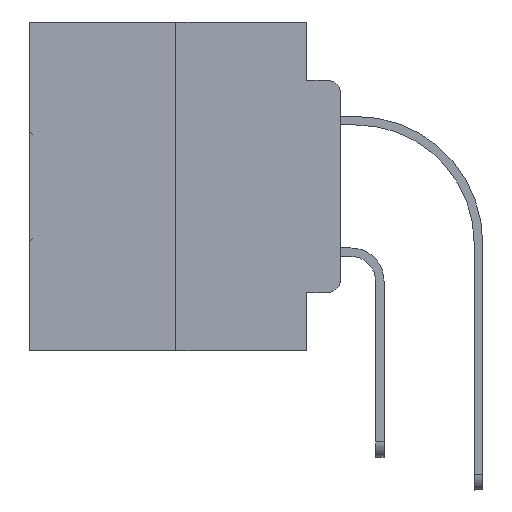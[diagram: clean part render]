
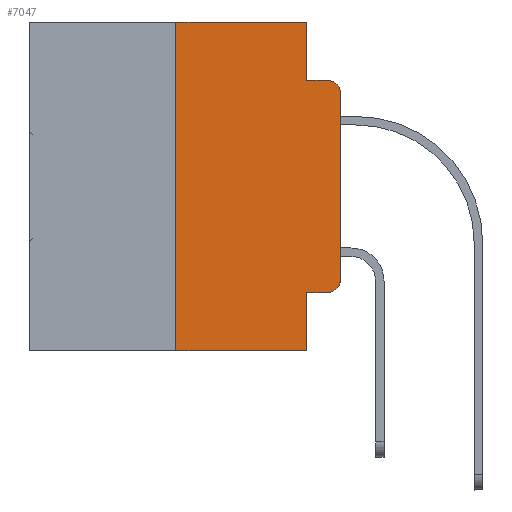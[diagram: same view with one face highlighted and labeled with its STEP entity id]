
A CAD part, left-side view. The second image highlights one B-rep face of the part: STEP entity #7047.
In plain terms, the highlighted planar face has unit normal (-1, 0, 0).
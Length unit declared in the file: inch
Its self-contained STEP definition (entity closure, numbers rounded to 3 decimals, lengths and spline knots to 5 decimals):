
#315 = EDGE_CURVE ( 'NONE', #3797, #12203, #30400, .T. ) ;
#463 = VECTOR ( 'NONE', #16938, 39.37008 ) ;
#603 = CARTESIAN_POINT ( 'NONE',  ( 0., 0.25, -0.5 ) ) ;
#805 = CARTESIAN_POINT ( 'NONE',  ( 0., 0.02, -0.1085 ) ) ;
#1443 = CARTESIAN_POINT ( 'NONE',  ( 0., 0.051, 0. ) ) ;
#1638 = CARTESIAN_POINT ( 'NONE',  ( 0., 0.25, 0. ) ) ;
#1700 = CARTESIAN_POINT ( 'NONE',  ( 0., 0.473, -0.5 ) ) ;
#1759 = ORIENTED_EDGE ( 'NONE', *, *, #17386, .F. ) ;
#2174 = LINE ( 'NONE', #17610, #9106 ) ;
#2386 = VECTOR ( 'NONE', #4438, 39.37008 ) ;
#3517 = LINE ( 'NONE', #11902, #11792 ) ;
#3520 = CARTESIAN_POINT ( 'NONE',  ( 0., 0.02, -0.0885 ) ) ;
#3797 = VERTEX_POINT ( 'NONE', #11076 ) ;
#4282 = LINE ( 'NONE', #1700, #2386 ) ;
#4438 = DIRECTION ( 'NONE',  ( 0., -1., 0. ) ) ;
#4453 = VECTOR ( 'NONE', #32825, 39.37008 ) ;
#4466 = EDGE_CURVE ( 'NONE', #33648, #27333, #4282, .T. ) ;
#5237 = CARTESIAN_POINT ( 'NONE',  ( 0., 0.051, -0.4115 ) ) ;
#5345 = DIRECTION ( 'NONE',  ( 0., 0., 1. ) ) ;
#5758 = VERTEX_POINT ( 'NONE', #30229 ) ;
#6590 = ORIENTED_EDGE ( 'NONE', *, *, #31161, .F. ) ;
#7047 = ADVANCED_FACE ( 'NONE', ( #12857 ), #25883, .F. ) ;
#8144 = EDGE_LOOP ( 'NONE', ( #18734, #12439, #12445, #6590, #8603, #12980, #22457, #1759, #18066, #11178 ) ) ;
#8603 = ORIENTED_EDGE ( 'NONE', *, *, #27772, .F. ) ;
#8847 = VECTOR ( 'NONE', #5345, 39.37008 ) ;
#9103 = CARTESIAN_POINT ( 'NONE',  ( 0., 0.051, 0. ) ) ;
#9106 = VECTOR ( 'NONE', #12625, 39.37008 ) ;
#9506 = AXIS2_PLACEMENT_3D ( 'NONE', #21875, #31980, #26991 ) ;
#10491 = LINE ( 'NONE', #28663, #8847 ) ;
#10568 = DIRECTION ( 'NONE',  ( 0., 0., 1. ) ) ;
#10963 = LINE ( 'NONE', #29975, #463 ) ;
#11076 = CARTESIAN_POINT ( 'NONE',  ( 0., 0., -0.1085 ) ) ;
#11178 = ORIENTED_EDGE ( 'NONE', *, *, #26241, .T. ) ;
#11747 = CARTESIAN_POINT ( 'NONE',  ( 0., 0.051, 0. ) ) ;
#11792 = VECTOR ( 'NONE', #29750, 39.37008 ) ;
#11902 = CARTESIAN_POINT ( 'NONE',  ( 0., 0.473, 0. ) ) ;
#12203 = VERTEX_POINT ( 'NONE', #3520 ) ;
#12439 = ORIENTED_EDGE ( 'NONE', *, *, #315, .T. ) ;
#12445 = ORIENTED_EDGE ( 'NONE', *, *, #13271, .F. ) ;
#12625 = DIRECTION ( 'NONE',  ( 0., -1., 0. ) ) ;
#12857 = FACE_OUTER_BOUND ( 'NONE', #8144, .T. ) ;
#12980 = ORIENTED_EDGE ( 'NONE', *, *, #29489, .F. ) ;
#13271 = EDGE_CURVE ( 'NONE', #13645, #12203, #10963, .T. ) ;
#13645 = VERTEX_POINT ( 'NONE', #31991 ) ;
#13906 = VERTEX_POINT ( 'NONE', #11747 ) ;
#14472 = LINE ( 'NONE', #1443, #4453 ) ;
#15547 = VERTEX_POINT ( 'NONE', #17035 ) ;
#16938 = DIRECTION ( 'NONE',  ( 0., -1., 0. ) ) ;
#17035 = CARTESIAN_POINT ( 'NONE',  ( 0., 0., -0.3915 ) ) ;
#17386 = EDGE_CURVE ( 'NONE', #33703, #27333, #14472, .T. ) ;
#17610 = CARTESIAN_POINT ( 'NONE',  ( 0., 0.051, -0.4115 ) ) ;
#18066 = ORIENTED_EDGE ( 'NONE', *, *, #30551, .T. ) ;
#18734 = ORIENTED_EDGE ( 'NONE', *, *, #20536, .T. ) ;
#19600 = DIRECTION ( 'NONE',  ( 0., 0., -1. ) ) ;
#20536 = EDGE_CURVE ( 'NONE', #15547, #3797, #10491, .T. ) ;
#21044 = LINE ( 'NONE', #26171, #23392 ) ;
#21792 = CARTESIAN_POINT ( 'NONE',  ( 0., 0.051, -0.5 ) ) ;
#21875 = CARTESIAN_POINT ( 'NONE',  ( 0., 0.02, -0.3915 ) ) ;
#22457 = ORIENTED_EDGE ( 'NONE', *, *, #4466, .T. ) ;
#22819 = DIRECTION ( 'NONE',  ( 1., 0., 0. ) ) ;
#23392 = VECTOR ( 'NONE', #10568, 39.37008 ) ;
#23962 = DIRECTION ( 'NONE',  ( -1., 0., 0. ) ) ;
#24623 = VERTEX_POINT ( 'NONE', #1638 ) ;
#25380 = DIRECTION ( 'NONE',  ( 0., 0., -1. ) ) ;
#25876 = VECTOR ( 'NONE', #19600, 39.37008 ) ;
#25883 = PLANE ( 'NONE',  #27819 ) ;
#25928 = CIRCLE ( 'NONE', #9506, 0.02 ) ;
#26171 = CARTESIAN_POINT ( 'NONE',  ( 0., 0.25, 0. ) ) ;
#26241 = EDGE_CURVE ( 'NONE', #5758, #15547, #25928, .T. ) ;
#26991 = DIRECTION ( 'NONE',  ( 0., 0., -1. ) ) ;
#27333 = VERTEX_POINT ( 'NONE', #21792 ) ;
#27646 = AXIS2_PLACEMENT_3D ( 'NONE', #805, #23962, #32179 ) ;
#27772 = EDGE_CURVE ( 'NONE', #24623, #13906, #3517, .T. ) ;
#27819 = AXIS2_PLACEMENT_3D ( 'NONE', #33618, #22819, #25380 ) ;
#28663 = CARTESIAN_POINT ( 'NONE',  ( 0., 0., 0. ) ) ;
#29489 = EDGE_CURVE ( 'NONE', #33648, #24623, #21044, .T. ) ;
#29750 = DIRECTION ( 'NONE',  ( 0., -1., 0. ) ) ;
#29975 = CARTESIAN_POINT ( 'NONE',  ( 0., 0.051, -0.0885 ) ) ;
#30229 = CARTESIAN_POINT ( 'NONE',  ( 0., 0.02, -0.4115 ) ) ;
#30400 = CIRCLE ( 'NONE', #27646, 0.02 ) ;
#30551 = EDGE_CURVE ( 'NONE', #33703, #5758, #2174, .T. ) ;
#31161 = EDGE_CURVE ( 'NONE', #13906, #13645, #32610, .T. ) ;
#31980 = DIRECTION ( 'NONE',  ( -1., 0., 0. ) ) ;
#31991 = CARTESIAN_POINT ( 'NONE',  ( 0., 0.051, -0.0885 ) ) ;
#32179 = DIRECTION ( 'NONE',  ( 0., 0., -1. ) ) ;
#32610 = LINE ( 'NONE', #9103, #25876 ) ;
#32825 = DIRECTION ( 'NONE',  ( 0., 0., -1. ) ) ;
#33618 = CARTESIAN_POINT ( 'NONE',  ( 0., 0.473, 0. ) ) ;
#33648 = VERTEX_POINT ( 'NONE', #603 ) ;
#33703 = VERTEX_POINT ( 'NONE', #5237 ) ;
